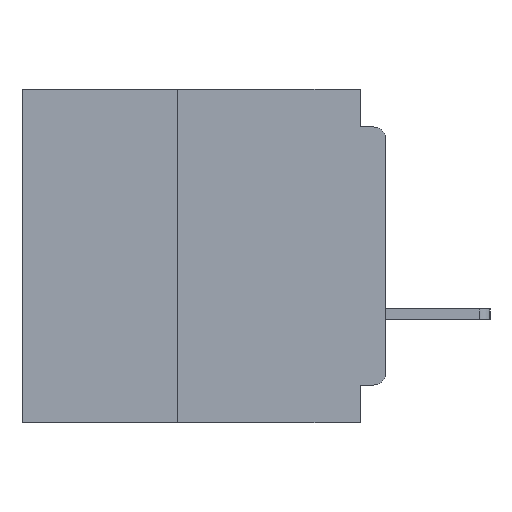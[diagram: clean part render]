
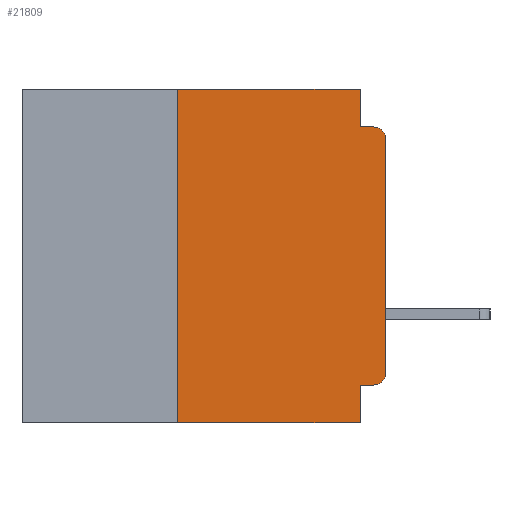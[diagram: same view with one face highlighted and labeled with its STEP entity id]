
A CAD part, left-side view. The second image highlights one B-rep face of the part: STEP entity #21809.
In plain terms, the highlighted planar face has unit normal (-1, 0, 0).
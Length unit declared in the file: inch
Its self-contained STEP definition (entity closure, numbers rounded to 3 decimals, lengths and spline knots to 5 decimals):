
#1086 = EDGE_CURVE ( 'NONE', #7919, #36755, #16247, .T. ) ;
#1605 = ORIENTED_EDGE ( 'NONE', *, *, #10759, .F. ) ;
#1756 = CARTESIAN_POINT ( 'NONE',  ( 0., 0.015, -0.355 ) ) ;
#1930 = CARTESIAN_POINT ( 'NONE',  ( 0., 0.437, 0. ) ) ;
#2473 = EDGE_CURVE ( 'NONE', #36755, #23820, #13302, .T. ) ;
#2524 = EDGE_CURVE ( 'NONE', #3902, #7919, #34550, .T. ) ;
#2715 = CARTESIAN_POINT ( 'NONE',  ( 0., 0.031, -0.4 ) ) ;
#3654 = EDGE_CURVE ( 'NONE', #23820, #36846, #25900, .T. ) ;
#3902 = VERTEX_POINT ( 'NONE', #22902 ) ;
#4687 = DIRECTION ( 'NONE',  ( 0., 0., 1. ) ) ;
#6746 = CARTESIAN_POINT ( 'NONE',  ( 0., 0., -0.045 ) ) ;
#6774 = VERTEX_POINT ( 'NONE', #9044 ) ;
#7180 = CARTESIAN_POINT ( 'NONE',  ( 0., 0.031, -0.355 ) ) ;
#7680 = ORIENTED_EDGE ( 'NONE', *, *, #26738, .F. ) ;
#7919 = VERTEX_POINT ( 'NONE', #26466 ) ;
#7971 = ORIENTED_EDGE ( 'NONE', *, *, #3654, .F. ) ;
#8928 = VECTOR ( 'NONE', #33594, 39.37008 ) ;
#9044 = CARTESIAN_POINT ( 'NONE',  ( 0., 0., -0.34 ) ) ;
#9471 = CARTESIAN_POINT ( 'NONE',  ( 0., 0., -0.06 ) ) ;
#9800 = DIRECTION ( 'NONE',  ( -1., 0., 0. ) ) ;
#10759 = EDGE_CURVE ( 'NONE', #30911, #13924, #24912, .T. ) ;
#11536 = ORIENTED_EDGE ( 'NONE', *, *, #2524, .F. ) ;
#12048 = CARTESIAN_POINT ( 'NONE',  ( 0., 0., -0.355 ) ) ;
#13302 = LINE ( 'NONE', #16084, #37387 ) ;
#13857 = DIRECTION ( 'NONE',  ( -1., 0., 0. ) ) ;
#13924 = VERTEX_POINT ( 'NONE', #2715 ) ;
#14555 = ORIENTED_EDGE ( 'NONE', *, *, #1086, .F. ) ;
#14739 = PLANE ( 'NONE',  #39011 ) ;
#14779 = CARTESIAN_POINT ( 'NONE',  ( 0., 0.031, 0. ) ) ;
#15300 = VECTOR ( 'NONE', #19965, 39.37008 ) ;
#15334 = FACE_OUTER_BOUND ( 'NONE', #23892, .T. ) ;
#15381 = CARTESIAN_POINT ( 'NONE',  ( 0., 0.031, -0.045 ) ) ;
#16084 = CARTESIAN_POINT ( 'NONE',  ( 0., 0.031, 0. ) ) ;
#16150 = VERTEX_POINT ( 'NONE', #1756 ) ;
#16247 = LINE ( 'NONE', #1930, #15300 ) ;
#16544 = VECTOR ( 'NONE', #18974, 39.37008 ) ;
#16869 = ORIENTED_EDGE ( 'NONE', *, *, #22241, .T. ) ;
#17736 = DIRECTION ( 'NONE',  ( 1., 0., 0. ) ) ;
#17877 = VECTOR ( 'NONE', #36972, 39.37008 ) ;
#18704 = CARTESIAN_POINT ( 'NONE',  ( 0., 0.015, -0.045 ) ) ;
#18752 = EDGE_CURVE ( 'NONE', #3902, #13924, #24497, .T. ) ;
#18971 = ORIENTED_EDGE ( 'NONE', *, *, #33481, .T. ) ;
#18974 = DIRECTION ( 'NONE',  ( 0., -1., 0. ) ) ;
#19965 = DIRECTION ( 'NONE',  ( 0., -1., 0. ) ) ;
#21215 = LINE ( 'NONE', #12048, #29276 ) ;
#21809 = ADVANCED_FACE ( 'NONE', ( #15334 ), #14739, .F. ) ;
#21998 = CARTESIAN_POINT ( 'NONE',  ( 0., 0.437, -0.4 ) ) ;
#22241 = EDGE_CURVE ( 'NONE', #6774, #29447, #35795, .T. ) ;
#22902 = CARTESIAN_POINT ( 'NONE',  ( 0., 0.25, -0.4 ) ) ;
#23820 = VERTEX_POINT ( 'NONE', #15381 ) ;
#23892 = EDGE_LOOP ( 'NONE', ( #16869, #18971, #7971, #37010, #14555, #11536, #36241, #1605, #7680, #32569 ) ) ;
#24497 = LINE ( 'NONE', #21998, #16544 ) ;
#24912 = LINE ( 'NONE', #27492, #8928 ) ;
#25900 = LINE ( 'NONE', #6746, #17877 ) ;
#26452 = VECTOR ( 'NONE', #34556, 39.37008 ) ;
#26466 = CARTESIAN_POINT ( 'NONE',  ( 0., 0.25, 0. ) ) ;
#26738 = EDGE_CURVE ( 'NONE', #16150, #30911, #21215, .T. ) ;
#26744 = VECTOR ( 'NONE', #4687, 39.37008 ) ;
#27360 = CIRCLE ( 'NONE', #33911, 0.015 ) ;
#27492 = CARTESIAN_POINT ( 'NONE',  ( 0., 0.031, -0.4 ) ) ;
#27822 = CARTESIAN_POINT ( 'NONE',  ( 0., 0.015, -0.06 ) ) ;
#28198 = DIRECTION ( 'NONE',  ( 0., 0., -1. ) ) ;
#28432 = CARTESIAN_POINT ( 'NONE',  ( 0., 0.25, -0.4 ) ) ;
#28659 = CIRCLE ( 'NONE', #31010, 0.015 ) ;
#28789 = CARTESIAN_POINT ( 'NONE',  ( 0., 0., 0. ) ) ;
#29276 = VECTOR ( 'NONE', #33138, 39.37008 ) ;
#29447 = VERTEX_POINT ( 'NONE', #9471 ) ;
#30865 = DIRECTION ( 'NONE',  ( 0., 0., -1. ) ) ;
#30911 = VERTEX_POINT ( 'NONE', #7180 ) ;
#31010 = AXIS2_PLACEMENT_3D ( 'NONE', #31931, #13857, #34982 ) ;
#31931 = CARTESIAN_POINT ( 'NONE',  ( 0., 0.015, -0.34 ) ) ;
#32569 = ORIENTED_EDGE ( 'NONE', *, *, #39189, .T. ) ;
#33138 = DIRECTION ( 'NONE',  ( 0., 1., 0. ) ) ;
#33481 = EDGE_CURVE ( 'NONE', #29447, #36846, #27360, .T. ) ;
#33594 = DIRECTION ( 'NONE',  ( 0., 0., -1. ) ) ;
#33911 = AXIS2_PLACEMENT_3D ( 'NONE', #27822, #9800, #30865 ) ;
#34550 = LINE ( 'NONE', #28432, #26452 ) ;
#34556 = DIRECTION ( 'NONE',  ( 0., 0., 1. ) ) ;
#34982 = DIRECTION ( 'NONE',  ( 0., 0., -1. ) ) ;
#35795 = LINE ( 'NONE', #28789, #26744 ) ;
#35861 = CARTESIAN_POINT ( 'NONE',  ( 0., 0.437, 0. ) ) ;
#36241 = ORIENTED_EDGE ( 'NONE', *, *, #18752, .T. ) ;
#36755 = VERTEX_POINT ( 'NONE', #14779 ) ;
#36846 = VERTEX_POINT ( 'NONE', #18704 ) ;
#36972 = DIRECTION ( 'NONE',  ( 0., -1., 0. ) ) ;
#37010 = ORIENTED_EDGE ( 'NONE', *, *, #2473, .F. ) ;
#37387 = VECTOR ( 'NONE', #28198, 39.37008 ) ;
#38883 = DIRECTION ( 'NONE',  ( 0., 0., -1. ) ) ;
#39011 = AXIS2_PLACEMENT_3D ( 'NONE', #35861, #17736, #38883 ) ;
#39189 = EDGE_CURVE ( 'NONE', #16150, #6774, #28659, .T. ) ;
